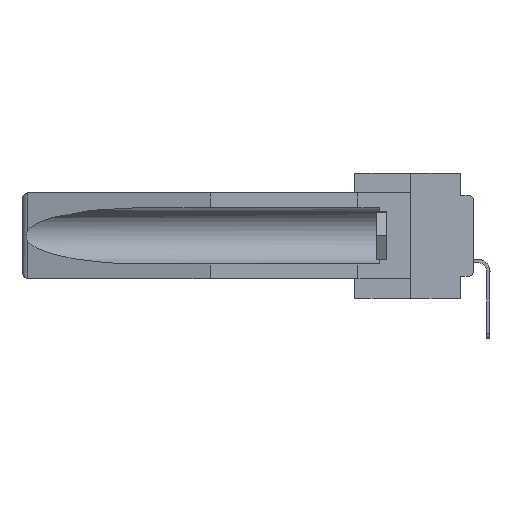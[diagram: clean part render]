
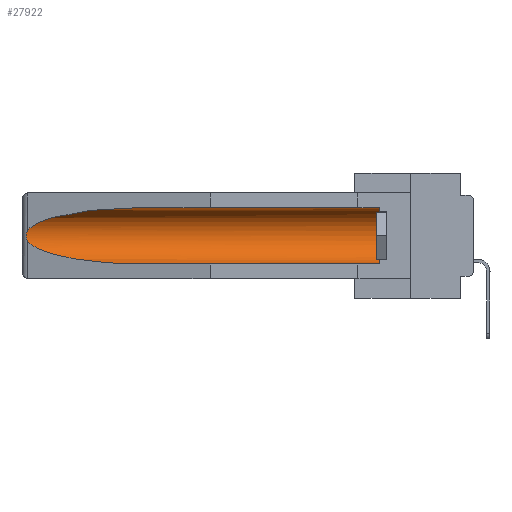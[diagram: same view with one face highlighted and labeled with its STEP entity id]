
A CAD part, left-side view. The second image highlights one B-rep face of the part: STEP entity #27922.
In plain terms, the highlighted cylindrical face has radius 2.857 mm (diameter 5.715 mm), a partial arc.
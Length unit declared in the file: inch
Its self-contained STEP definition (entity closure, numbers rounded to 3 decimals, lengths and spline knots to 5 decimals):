
#297 = CYLINDRICAL_SURFACE ( 'NONE', #30131, 0.1125 ) ;
#303 = CARTESIAN_POINT ( 'NONE',  ( 0.25451, 1.48313, -0.24835 ) ) ;
#506 = CARTESIAN_POINT ( 'NONE',  ( 0.26537, 1.52718, -0.14972 ) ) ;
#874 = EDGE_CURVE ( 'NONE', #18492, #21626, #11361, .T. ) ;
#1082 = AXIS2_PLACEMENT_3D ( 'NONE', #5399, #7654, #24779 ) ;
#1623 = EDGE_CURVE ( 'NONE', #21626, #30367, #31604, .T. ) ;
#2541 = DIRECTION ( 'NONE',  ( 0., 0., 1. ) ) ;
#2705 = CARTESIAN_POINT ( 'NONE',  ( 0.26537, 1.52718, -0.19328 ) ) ;
#2818 = CARTESIAN_POINT ( 'NONE',  ( 0.26655, 1.53094, -0.18657 ) ) ;
#2922 = ORIENTED_EDGE ( 'NONE', *, *, #29500, .T. ) ;
#3020 = LINE ( 'NONE', #3341, #15140 ) ;
#3341 = CARTESIAN_POINT ( 'NONE',  ( 0.155, -0.30754, -0.284 ) ) ;
#4096 = EDGE_LOOP ( 'NONE', ( #9228, #27440, #19704, #25537, #24522, #2922 ) ) ;
#4313 = CARTESIAN_POINT ( 'NONE',  ( 0.155, 1.07973, -0.059 ) ) ;
#4912 = VERTEX_POINT ( 'NONE', #30266 ) ;
#5399 = CARTESIAN_POINT ( 'NONE',  ( 0.155, 0.126, -0.1715 ) ) ;
#5585 =( BOUNDED_CURVE ( )  B_SPLINE_CURVE ( 3, ( #2705, #303, #27631, #15324 ),
 .UNSPECIFIED., .F., .F. ) 
 B_SPLINE_CURVE_WITH_KNOTS ( ( 4, 4 ),
 ( 0.1948, 1.5708 ),
 .UNSPECIFIED. ) 
 CURVE ( )  GEOMETRIC_REPRESENTATION_ITEM ( )  RATIONAL_B_SPLINE_CURVE ( ( 1., 0.848, 0.848, 1. ) ) 
 REPRESENTATION_ITEM ( '' )  );
#5698 = CARTESIAN_POINT ( 'NONE',  ( 0.2675, 1.53308, -0.16763 ) ) ;
#6242 = CIRCLE ( 'NONE', #1082, 0.1125 ) ;
#7133 = EDGE_CURVE ( 'NONE', #31280, #4912, #6242, .T. ) ;
#7654 = DIRECTION ( 'NONE',  ( 0., -1., 0. ) ) ;
#8246 = CARTESIAN_POINT ( 'NONE',  ( 0.26537, 1.52718, -0.14972 ) ) ;
#9228 = ORIENTED_EDGE ( 'NONE', *, *, #874, .T. ) ;
#9827 = FACE_OUTER_BOUND ( 'NONE', #4096, .T. ) ;
#10682 = VERTEX_POINT ( 'NONE', #19211 ) ;
#10740 = CARTESIAN_POINT ( 'NONE',  ( 0.26537, 1.52718, -0.14972 ) ) ;
#11361 =( BOUNDED_CURVE ( )  B_SPLINE_CURVE ( 3, ( #4313, #20692, #11771, #8246 ),
 .UNSPECIFIED., .F., .F. ) 
 B_SPLINE_CURVE_WITH_KNOTS ( ( 4, 4 ),
 ( 4.71239, 6.08839 ),
 .UNSPECIFIED. ) 
 CURVE ( )  GEOMETRIC_REPRESENTATION_ITEM ( )  RATIONAL_B_SPLINE_CURVE ( ( 1., 0.848, 0.848, 1. ) ) 
 REPRESENTATION_ITEM ( '' )  );
#11771 = CARTESIAN_POINT ( 'NONE',  ( 0.25451, 1.48313, -0.09465 ) ) ;
#12660 = CARTESIAN_POINT ( 'NONE',  ( 0.155, -0.30754, -0.059 ) ) ;
#12697 = CARTESIAN_POINT ( 'NONE',  ( 0.2673, 1.53269, -0.17917 ) ) ;
#14628 = CARTESIAN_POINT ( 'NONE',  ( 0.26537, 1.52718, -0.19328 ) ) ;
#15140 = VECTOR ( 'NONE', #30205, 39.37008 ) ;
#15324 = CARTESIAN_POINT ( 'NONE',  ( 0.155, 1.07973, -0.284 ) ) ;
#16269 = VECTOR ( 'NONE', #29310, 39.37008 ) ;
#16280 = CARTESIAN_POINT ( 'NONE',  ( 0.155, 1.07973, -0.059 ) ) ;
#17669 = CARTESIAN_POINT ( 'NONE',  ( 0.2675, 1.53308, -0.17534 ) ) ;
#18492 = VERTEX_POINT ( 'NONE', #16280 ) ;
#19211 = CARTESIAN_POINT ( 'NONE',  ( 0.155, 1.07973, -0.284 ) ) ;
#19675 = CARTESIAN_POINT ( 'NONE',  ( 0.155, -0.30754, -0.1715 ) ) ;
#19704 = ORIENTED_EDGE ( 'NONE', *, *, #28859, .T. ) ;
#20433 = CARTESIAN_POINT ( 'NONE',  ( 0.2673, 1.5327, -0.16383 ) ) ;
#20692 = CARTESIAN_POINT ( 'NONE',  ( 0.21114, 1.30732, -0.059 ) ) ;
#21626 = VERTEX_POINT ( 'NONE', #506 ) ;
#22529 = CARTESIAN_POINT ( 'NONE',  ( 0.26537, 1.52718, -0.19328 ) ) ;
#22843 = CARTESIAN_POINT ( 'NONE',  ( 0.26654, 1.53092, -0.15636 ) ) ;
#24522 = ORIENTED_EDGE ( 'NONE', *, *, #7133, .T. ) ;
#24779 = DIRECTION ( 'NONE',  ( 0., 0., 1. ) ) ;
#25125 = CARTESIAN_POINT ( 'NONE',  ( 0.26597, 1.52961, -0.15275 ) ) ;
#25528 = CARTESIAN_POINT ( 'NONE',  ( 0.155, 0.126, -0.284 ) ) ;
#25537 = ORIENTED_EDGE ( 'NONE', *, *, #28066, .F. ) ;
#27135 = DIRECTION ( 'NONE',  ( 0., 1., 0. ) ) ;
#27440 = ORIENTED_EDGE ( 'NONE', *, *, #1623, .T. ) ;
#27631 = CARTESIAN_POINT ( 'NONE',  ( 0.21114, 1.30732, -0.284 ) ) ;
#27922 = ADVANCED_FACE ( 'NONE', ( #9827 ), #297, .F. ) ;
#28066 = EDGE_CURVE ( 'NONE', #31280, #10682, #3020, .T. ) ;
#28859 = EDGE_CURVE ( 'NONE', #30367, #10682, #5585, .T. ) ;
#29310 = DIRECTION ( 'NONE',  ( 0., 1., 0. ) ) ;
#29500 = EDGE_CURVE ( 'NONE', #4912, #18492, #31896, .T. ) ;
#29979 = CARTESIAN_POINT ( 'NONE',  ( 0.26597, 1.5296, -0.19026 ) ) ;
#30131 = AXIS2_PLACEMENT_3D ( 'NONE', #19675, #27135, #2541 ) ;
#30205 = DIRECTION ( 'NONE',  ( 0., 1., 0. ) ) ;
#30266 = CARTESIAN_POINT ( 'NONE',  ( 0.155, 0.126, -0.059 ) ) ;
#30367 = VERTEX_POINT ( 'NONE', #14628 ) ;
#31280 = VERTEX_POINT ( 'NONE', #25528 ) ;
#31604 = B_SPLINE_CURVE_WITH_KNOTS ( 'NONE', 3,
 ( #10740, #25125, #22843, #20433, #5698, #17669, #12697, #2818, #29979, #22529 ),
 .UNSPECIFIED., .F., .F.,
 ( 4, 2, 2, 2, 4 ),
 ( 0., 0.00029, 0.00058, 0.00087, 0.00117 ),
 .UNSPECIFIED. ) ;
#31896 = LINE ( 'NONE', #12660, #16269 ) ;
